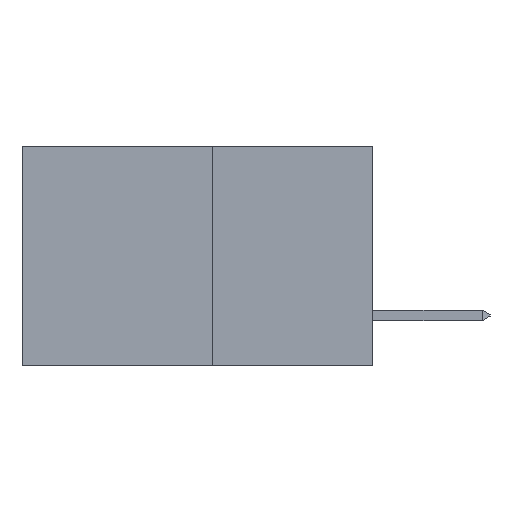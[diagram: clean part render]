
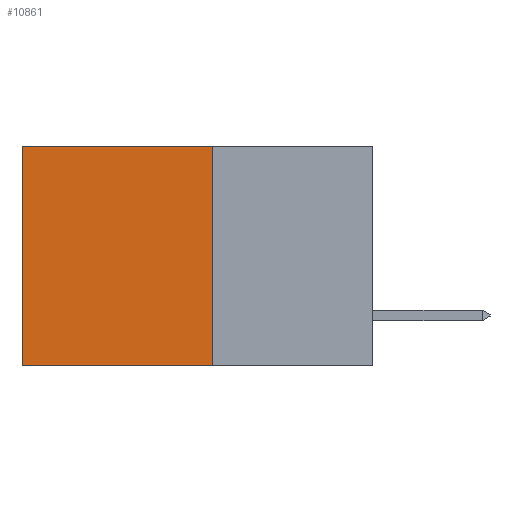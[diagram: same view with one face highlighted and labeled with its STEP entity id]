
A CAD part, left-side view. The second image highlights one B-rep face of the part: STEP entity #10861.
In plain terms, the highlighted planar face has unit normal (-1, 0, 0).
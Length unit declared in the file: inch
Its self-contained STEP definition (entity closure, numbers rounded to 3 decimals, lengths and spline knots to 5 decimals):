
#885 = LINE ( 'NONE', #16177, #20646 ) ;
#1346 = VERTEX_POINT ( 'NONE', #11036 ) ;
#1370 = ORIENTED_EDGE ( 'NONE', *, *, #18643, .T. ) ;
#2984 = CARTESIAN_POINT ( 'NONE',  ( 0.277, 0.27, -0.37 ) ) ;
#3636 = ORIENTED_EDGE ( 'NONE', *, *, #10360, .F. ) ;
#4139 = LINE ( 'NONE', #2984, #13459 ) ;
#5745 = CARTESIAN_POINT ( 'NONE',  ( 0.277, 0.59, -0.37 ) ) ;
#6252 = CARTESIAN_POINT ( 'NONE',  ( 0.277, 0.27, 0. ) ) ;
#6627 = PLANE ( 'NONE',  #17483 ) ;
#6950 = CARTESIAN_POINT ( 'NONE',  ( 0.277, 0.27, -0.37 ) ) ;
#9357 = VECTOR ( 'NONE', #20541, 39.37008 ) ;
#10360 = EDGE_CURVE ( 'NONE', #15208, #1346, #885, .T. ) ;
#10414 = CARTESIAN_POINT ( 'NONE',  ( 0.277, 0.27, -0.37 ) ) ;
#10861 = ADVANCED_FACE ( 'NONE', ( #13398 ), #6627, .F. ) ;
#11036 = CARTESIAN_POINT ( 'NONE',  ( 0.277, 0.59, -0.37 ) ) ;
#12068 = CARTESIAN_POINT ( 'NONE',  ( 0.277, 0.59, 0. ) ) ;
#12253 = DIRECTION ( 'NONE',  ( 0., 0., -1. ) ) ;
#13107 = ORIENTED_EDGE ( 'NONE', *, *, #15139, .F. ) ;
#13149 = CARTESIAN_POINT ( 'NONE',  ( 0.277, 0.27, 0. ) ) ;
#13398 = FACE_OUTER_BOUND ( 'NONE', #13745, .T. ) ;
#13459 = VECTOR ( 'NONE', #23310, 39.37008 ) ;
#13745 = EDGE_LOOP ( 'NONE', ( #1370, #3636, #13107, #17888 ) ) ;
#14205 = LINE ( 'NONE', #5745, #9357 ) ;
#14209 = VERTEX_POINT ( 'NONE', #13149 ) ;
#15139 = EDGE_CURVE ( 'NONE', #14209, #15208, #4139, .T. ) ;
#15208 = VERTEX_POINT ( 'NONE', #6950 ) ;
#15374 = LINE ( 'NONE', #6252, #20891 ) ;
#16177 = CARTESIAN_POINT ( 'NONE',  ( 0.277, 0.27, -0.37 ) ) ;
#17483 = AXIS2_PLACEMENT_3D ( 'NONE', #10414, #23235, #12253 ) ;
#17888 = ORIENTED_EDGE ( 'NONE', *, *, #18153, .T. ) ;
#18153 = EDGE_CURVE ( 'NONE', #14209, #22497, #15374, .T. ) ;
#18643 = EDGE_CURVE ( 'NONE', #22497, #1346, #14205, .T. ) ;
#19125 = DIRECTION ( 'NONE',  ( 0., 1., 0. ) ) ;
#20541 = DIRECTION ( 'NONE',  ( 0., 0., -1. ) ) ;
#20646 = VECTOR ( 'NONE', #21674, 39.37008 ) ;
#20891 = VECTOR ( 'NONE', #19125, 39.37008 ) ;
#21674 = DIRECTION ( 'NONE',  ( 0., 1., 0. ) ) ;
#22497 = VERTEX_POINT ( 'NONE', #12068 ) ;
#23235 = DIRECTION ( 'NONE',  ( 1., 0., 0. ) ) ;
#23310 = DIRECTION ( 'NONE',  ( 0., 0., -1. ) ) ;
